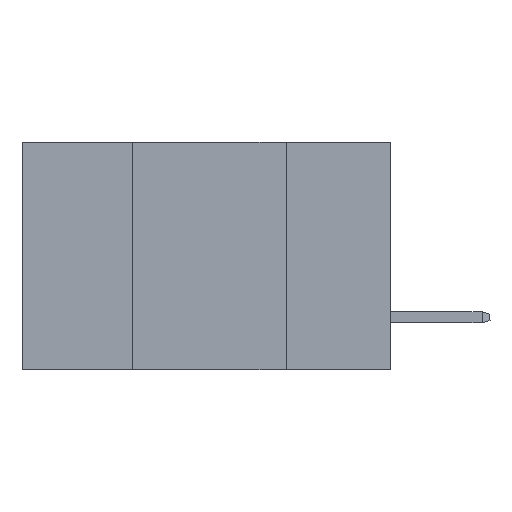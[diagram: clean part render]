
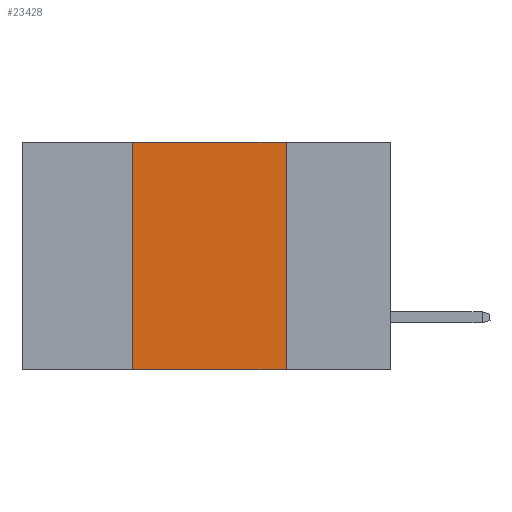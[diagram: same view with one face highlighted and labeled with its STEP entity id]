
A CAD part, left-side view. The second image highlights one B-rep face of the part: STEP entity #23428.
In plain terms, the highlighted planar face has unit normal (-1, 0, 0).
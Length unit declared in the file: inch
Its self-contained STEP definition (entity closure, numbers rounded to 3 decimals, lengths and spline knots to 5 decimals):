
#634 = DIRECTION ( 'NONE',  ( 0., 0., -1. ) ) ;
#677 = DIRECTION ( 'NONE',  ( 0., 0., 1. ) ) ;
#2882 = CARTESIAN_POINT ( 'NONE',  ( 0., 0.42, 0. ) ) ;
#3069 = PLANE ( 'NONE',  #11792 ) ;
#3251 = ORIENTED_EDGE ( 'NONE', *, *, #14228, .F. ) ;
#3702 = VERTEX_POINT ( 'NONE', #25549 ) ;
#5233 = CARTESIAN_POINT ( 'NONE',  ( 0., 0.17, 0. ) ) ;
#5375 = CARTESIAN_POINT ( 'NONE',  ( 0., 0.6, 0. ) ) ;
#6855 = VERTEX_POINT ( 'NONE', #25132 ) ;
#7231 = ORIENTED_EDGE ( 'NONE', *, *, #15425, .F. ) ;
#7568 = FACE_OUTER_BOUND ( 'NONE', #19000, .T. ) ;
#7706 = DIRECTION ( 'NONE',  ( 1., 0., 0. ) ) ;
#10875 = CARTESIAN_POINT ( 'NONE',  ( 0., 0.6, -0.37 ) ) ;
#11792 = AXIS2_PLACEMENT_3D ( 'NONE', #5375, #7706, #23984 ) ;
#12046 = EDGE_CURVE ( 'NONE', #6855, #3702, #19325, .T. ) ;
#13065 = ORIENTED_EDGE ( 'NONE', *, *, #21007, .T. ) ;
#13166 = VECTOR ( 'NONE', #634, 39.37008 ) ;
#13235 = DIRECTION ( 'NONE',  ( 0., -1., 0. ) ) ;
#13685 = CARTESIAN_POINT ( 'NONE',  ( 0., 0.42, 0. ) ) ;
#13769 = LINE ( 'NONE', #2882, #25372 ) ;
#13888 = VECTOR ( 'NONE', #13235, 39.37008 ) ;
#14228 = EDGE_CURVE ( 'NONE', #14478, #17547, #13769, .T. ) ;
#14342 = VECTOR ( 'NONE', #21470, 39.37008 ) ;
#14478 = VERTEX_POINT ( 'NONE', #15462 ) ;
#15425 = EDGE_CURVE ( 'NONE', #17547, #6855, #27390, .T. ) ;
#15462 = CARTESIAN_POINT ( 'NONE',  ( 0., 0.42, -0.37 ) ) ;
#17547 = VERTEX_POINT ( 'NONE', #13685 ) ;
#18163 = ORIENTED_EDGE ( 'NONE', *, *, #12046, .F. ) ;
#19000 = EDGE_LOOP ( 'NONE', ( #18163, #7231, #3251, #13065 ) ) ;
#19325 = LINE ( 'NONE', #5233, #13166 ) ;
#21007 = EDGE_CURVE ( 'NONE', #14478, #3702, #26208, .T. ) ;
#21470 = DIRECTION ( 'NONE',  ( 0., -1., 0. ) ) ;
#23428 = ADVANCED_FACE ( 'NONE', ( #7568 ), #3069, .F. ) ;
#23984 = DIRECTION ( 'NONE',  ( 0., 0., -1. ) ) ;
#25132 = CARTESIAN_POINT ( 'NONE',  ( 0., 0.17, 0. ) ) ;
#25372 = VECTOR ( 'NONE', #677, 39.37008 ) ;
#25549 = CARTESIAN_POINT ( 'NONE',  ( 0., 0.17, -0.37 ) ) ;
#26055 = CARTESIAN_POINT ( 'NONE',  ( 0., 0.6, 0. ) ) ;
#26208 = LINE ( 'NONE', #10875, #13888 ) ;
#27390 = LINE ( 'NONE', #26055, #14342 ) ;
